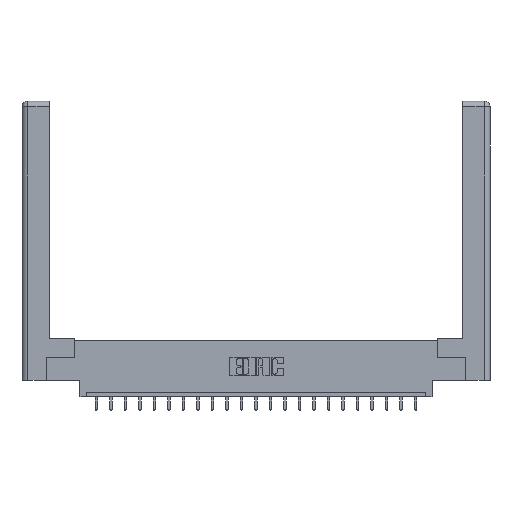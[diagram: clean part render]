
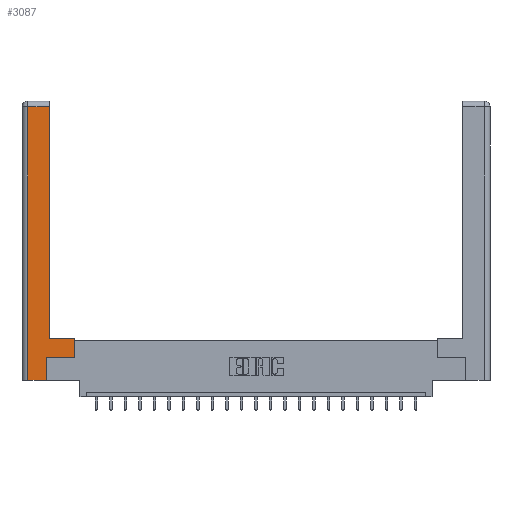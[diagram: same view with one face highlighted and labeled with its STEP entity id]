
A CAD part, top view. The second image highlights one B-rep face of the part: STEP entity #3087.
In plain terms, the highlighted planar face has unit normal (0, 0, 1).
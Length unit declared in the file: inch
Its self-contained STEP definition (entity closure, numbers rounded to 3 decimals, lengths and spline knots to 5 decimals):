
#432 = CARTESIAN_POINT ( 'NONE',  ( 0.565, 0.245, 0. ) ) ;
#473 = LINE ( 'NONE', #8664, #21985 ) ;
#532 = CARTESIAN_POINT ( 'NONE',  ( 0.565, 0.45, 0. ) ) ;
#706 = EDGE_LOOP ( 'NONE', ( #8781, #8390, #17514, #9704, #2646, #12398, #1213, #7319 ) ) ;
#1090 = VECTOR ( 'NONE', #17355, 39.37008 ) ;
#1213 = ORIENTED_EDGE ( 'NONE', *, *, #18896, .T. ) ;
#1731 = CARTESIAN_POINT ( 'NONE',  ( 0.265, 0., 0. ) ) ;
#1927 = FACE_OUTER_BOUND ( 'NONE', #706, .T. ) ;
#1945 = VERTEX_POINT ( 'NONE', #2926 ) ;
#2547 = EDGE_CURVE ( 'NONE', #11229, #5239, #6005, .T. ) ;
#2646 = ORIENTED_EDGE ( 'NONE', *, *, #2547, .T. ) ;
#2926 = CARTESIAN_POINT ( 'NONE',  ( 0.0615, 0., 0. ) ) ;
#3087 = ADVANCED_FACE ( 'NONE', ( #1927 ), #15236, .F. ) ;
#3340 = EDGE_CURVE ( 'NONE', #1945, #11229, #14799, .T. ) ;
#3373 = CARTESIAN_POINT ( 'NONE',  ( 0.295, 3., 0. ) ) ;
#3703 = VERTEX_POINT ( 'NONE', #432 ) ;
#4009 = DIRECTION ( 'NONE',  ( 0., 1., 0. ) ) ;
#4167 = CARTESIAN_POINT ( 'NONE',  ( 0.0615, 2.94, 0. ) ) ;
#4617 = EDGE_CURVE ( 'NONE', #10046, #22128, #15017, .T. ) ;
#5076 = CARTESIAN_POINT ( 'NONE',  ( 0.0615, 0., 0. ) ) ;
#5237 = DIRECTION ( 'NONE',  ( -1., 0., 0. ) ) ;
#5239 = VERTEX_POINT ( 'NONE', #6649 ) ;
#5475 = CARTESIAN_POINT ( 'NONE',  ( 0.265, 0., 0. ) ) ;
#5796 = VECTOR ( 'NONE', #15145, 39.37008 ) ;
#5935 = VECTOR ( 'NONE', #20644, 39.37008 ) ;
#6005 = LINE ( 'NONE', #11373, #12962 ) ;
#6295 = CARTESIAN_POINT ( 'NONE',  ( 0.295, 2.94, 0. ) ) ;
#6649 = CARTESIAN_POINT ( 'NONE',  ( 0.265, 0.245, 0. ) ) ;
#6825 = CARTESIAN_POINT ( 'NONE',  ( 0.565, 0.45, 0. ) ) ;
#6855 = DIRECTION ( 'NONE',  ( 0., 0., -1. ) ) ;
#6954 = CARTESIAN_POINT ( 'NONE',  ( 0.295, 0.45, 0. ) ) ;
#7319 = ORIENTED_EDGE ( 'NONE', *, *, #4617, .T. ) ;
#7808 = DIRECTION ( 'NONE',  ( 0., 1., 0. ) ) ;
#8066 = EDGE_CURVE ( 'NONE', #22128, #19234, #10346, .T. ) ;
#8390 = ORIENTED_EDGE ( 'NONE', *, *, #14207, .T. ) ;
#8664 = CARTESIAN_POINT ( 'NONE',  ( 0.565, 0.245, 0. ) ) ;
#8781 = ORIENTED_EDGE ( 'NONE', *, *, #8066, .T. ) ;
#9704 = ORIENTED_EDGE ( 'NONE', *, *, #3340, .T. ) ;
#9874 = VECTOR ( 'NONE', #5237, 39.37008 ) ;
#9982 = LINE ( 'NONE', #5076, #20775 ) ;
#10046 = VERTEX_POINT ( 'NONE', #6825 ) ;
#10346 = LINE ( 'NONE', #3373, #5796 ) ;
#11229 = VERTEX_POINT ( 'NONE', #1731 ) ;
#11373 = CARTESIAN_POINT ( 'NONE',  ( 0.265, 0.245, 0. ) ) ;
#12058 = CARTESIAN_POINT ( 'NONE',  ( 0.0615, 2.94, 0. ) ) ;
#12191 = AXIS2_PLACEMENT_3D ( 'NONE', #20323, #6855, #15318 ) ;
#12384 = EDGE_CURVE ( 'NONE', #21944, #1945, #9982, .T. ) ;
#12398 = ORIENTED_EDGE ( 'NONE', *, *, #17603, .T. ) ;
#12962 = VECTOR ( 'NONE', #7808, 39.37008 ) ;
#13320 = CARTESIAN_POINT ( 'NONE',  ( 0.295, 0.45, 0. ) ) ;
#13601 = VECTOR ( 'NONE', #4009, 39.37008 ) ;
#14207 = EDGE_CURVE ( 'NONE', #19234, #21944, #17984, .T. ) ;
#14799 = LINE ( 'NONE', #5475, #1090 ) ;
#15017 = LINE ( 'NONE', #6954, #5935 ) ;
#15145 = DIRECTION ( 'NONE',  ( 0., 1., 0. ) ) ;
#15236 = PLANE ( 'NONE',  #12191 ) ;
#15318 = DIRECTION ( 'NONE',  ( -1., 0., 0. ) ) ;
#17355 = DIRECTION ( 'NONE',  ( 1., 0., 0. ) ) ;
#17424 = DIRECTION ( 'NONE',  ( 0., -1., 0. ) ) ;
#17514 = ORIENTED_EDGE ( 'NONE', *, *, #12384, .T. ) ;
#17603 = EDGE_CURVE ( 'NONE', #5239, #3703, #473, .T. ) ;
#17984 = LINE ( 'NONE', #12058, #9874 ) ;
#18725 = DIRECTION ( 'NONE',  ( 1., 0., 0. ) ) ;
#18896 = EDGE_CURVE ( 'NONE', #3703, #10046, #20965, .T. ) ;
#19234 = VERTEX_POINT ( 'NONE', #6295 ) ;
#20323 = CARTESIAN_POINT ( 'NONE',  ( 0., 0., 0. ) ) ;
#20644 = DIRECTION ( 'NONE',  ( -1., 0., 0. ) ) ;
#20775 = VECTOR ( 'NONE', #17424, 39.37008 ) ;
#20965 = LINE ( 'NONE', #532, #13601 ) ;
#21944 = VERTEX_POINT ( 'NONE', #4167 ) ;
#21985 = VECTOR ( 'NONE', #18725, 39.37008 ) ;
#22128 = VERTEX_POINT ( 'NONE', #13320 ) ;
